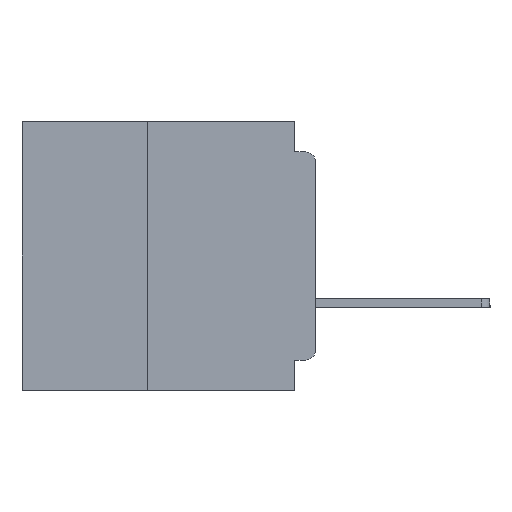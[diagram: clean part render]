
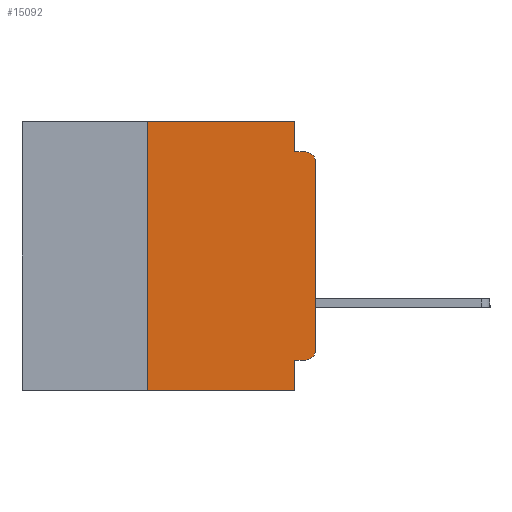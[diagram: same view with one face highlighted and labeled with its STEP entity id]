
A CAD part, left-side view. The second image highlights one B-rep face of the part: STEP entity #15092.
In plain terms, the highlighted planar face has unit normal (-1, 0, 0).
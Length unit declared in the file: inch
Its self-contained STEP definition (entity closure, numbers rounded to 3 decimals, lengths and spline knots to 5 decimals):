
#999 = VERTEX_POINT ( 'NONE', #19399 ) ;
#2351 = VECTOR ( 'NONE', #28648, 39.37008 ) ;
#2496 = EDGE_CURVE ( 'NONE', #19517, #46442, #31707, .T. ) ;
#2629 = VECTOR ( 'NONE', #43615, 39.37008 ) ;
#3094 = DIRECTION ( 'NONE',  ( 1., 0., 0. ) ) ;
#3157 = VERTEX_POINT ( 'NONE', #3941 ) ;
#3846 = DIRECTION ( 'NONE',  ( 0., -1., 0. ) ) ;
#3941 = CARTESIAN_POINT ( 'NONE',  ( 0., 0.031, -0.4 ) ) ;
#4085 = CARTESIAN_POINT ( 'NONE',  ( 0., 0.031, -0.4 ) ) ;
#4223 = CIRCLE ( 'NONE', #15329, 0.015 ) ;
#4745 = AXIS2_PLACEMENT_3D ( 'NONE', #50031, #23268, #54496 ) ;
#5116 = FACE_OUTER_BOUND ( 'NONE', #40707, .T. ) ;
#6350 = ORIENTED_EDGE ( 'NONE', *, *, #2496, .F. ) ;
#6652 = CARTESIAN_POINT ( 'NONE',  ( 0., 0.25, 0. ) ) ;
#7062 = ORIENTED_EDGE ( 'NONE', *, *, #38648, .F. ) ;
#8152 = EDGE_CURVE ( 'NONE', #999, #46442, #39294, .T. ) ;
#9086 = VERTEX_POINT ( 'NONE', #50397 ) ;
#9133 = ORIENTED_EDGE ( 'NONE', *, *, #21277, .T. ) ;
#10361 = ORIENTED_EDGE ( 'NONE', *, *, #40444, .F. ) ;
#11088 = VERTEX_POINT ( 'NONE', #11302 ) ;
#11302 = CARTESIAN_POINT ( 'NONE',  ( 0., 0.031, 0. ) ) ;
#12837 = CARTESIAN_POINT ( 'NONE',  ( 0., 0.437, -0.4 ) ) ;
#14018 = VECTOR ( 'NONE', #33196, 39.37008 ) ;
#14271 = LINE ( 'NONE', #41947, #2351 ) ;
#14731 = DIRECTION ( 'NONE',  ( 0., 0., 1. ) ) ;
#15092 = ADVANCED_FACE ( 'NONE', ( #5116 ), #25360, .F. ) ;
#15226 = CARTESIAN_POINT ( 'NONE',  ( 0., 0., -0.355 ) ) ;
#15329 = AXIS2_PLACEMENT_3D ( 'NONE', #21290, #52503, #25749 ) ;
#15903 = LINE ( 'NONE', #46033, #39646 ) ;
#18441 = VECTOR ( 'NONE', #56700, 39.37008 ) ;
#19144 = ORIENTED_EDGE ( 'NONE', *, *, #37119, .F. ) ;
#19195 = LINE ( 'NONE', #4085, #53429 ) ;
#19399 = CARTESIAN_POINT ( 'NONE',  ( 0., 0., -0.06 ) ) ;
#19517 = VERTEX_POINT ( 'NONE', #54055 ) ;
#20667 = VERTEX_POINT ( 'NONE', #41585 ) ;
#21005 = CARTESIAN_POINT ( 'NONE',  ( 0., 0., -0.045 ) ) ;
#21277 = EDGE_CURVE ( 'NONE', #20667, #999, #15903, .T. ) ;
#21290 = CARTESIAN_POINT ( 'NONE',  ( 0., 0.015, -0.34 ) ) ;
#22080 = CARTESIAN_POINT ( 'NONE',  ( 0., 0.015, -0.355 ) ) ;
#23118 = VECTOR ( 'NONE', #3846, 39.37008 ) ;
#23268 = DIRECTION ( 'NONE',  ( -1., 0., 0. ) ) ;
#25360 = PLANE ( 'NONE',  #29732 ) ;
#25749 = DIRECTION ( 'NONE',  ( 0., 0., -1. ) ) ;
#25896 = LINE ( 'NONE', #15226, #14018 ) ;
#28648 = DIRECTION ( 'NONE',  ( 0., 0., 1. ) ) ;
#28824 = VERTEX_POINT ( 'NONE', #46643 ) ;
#29732 = AXIS2_PLACEMENT_3D ( 'NONE', #56581, #3094, #34353 ) ;
#31707 = LINE ( 'NONE', #21005, #18441 ) ;
#33194 = ORIENTED_EDGE ( 'NONE', *, *, #40714, .F. ) ;
#33196 = DIRECTION ( 'NONE',  ( 0., 1., 0. ) ) ;
#33329 = DIRECTION ( 'NONE',  ( 0., -1., 0. ) ) ;
#34353 = DIRECTION ( 'NONE',  ( 0., 0., -1. ) ) ;
#34751 = LINE ( 'NONE', #55386, #45253 ) ;
#35011 = LINE ( 'NONE', #12837, #23118 ) ;
#35567 = VERTEX_POINT ( 'NONE', #6652 ) ;
#36502 = ORIENTED_EDGE ( 'NONE', *, *, #37325, .T. ) ;
#37119 = EDGE_CURVE ( 'NONE', #51397, #9086, #25896, .T. ) ;
#37325 = EDGE_CURVE ( 'NONE', #51397, #20667, #4223, .T. ) ;
#38648 = EDGE_CURVE ( 'NONE', #11088, #19517, #48793, .T. ) ;
#39294 = CIRCLE ( 'NONE', #4745, 0.015 ) ;
#39646 = VECTOR ( 'NONE', #14731, 39.37008 ) ;
#40444 = EDGE_CURVE ( 'NONE', #9086, #3157, #19195, .T. ) ;
#40707 = EDGE_LOOP ( 'NONE', ( #9133, #46106, #6350, #7062, #42243, #33194, #49596, #10361, #19144, #36502 ) ) ;
#40714 = EDGE_CURVE ( 'NONE', #28824, #35567, #14271, .T. ) ;
#41585 = CARTESIAN_POINT ( 'NONE',  ( 0., 0., -0.34 ) ) ;
#41947 = CARTESIAN_POINT ( 'NONE',  ( 0., 0.25, -0.4 ) ) ;
#42243 = ORIENTED_EDGE ( 'NONE', *, *, #42609, .F. ) ;
#42609 = EDGE_CURVE ( 'NONE', #35567, #11088, #34751, .T. ) ;
#43615 = DIRECTION ( 'NONE',  ( 0., 0., -1. ) ) ;
#45253 = VECTOR ( 'NONE', #33329, 39.37008 ) ;
#46033 = CARTESIAN_POINT ( 'NONE',  ( 0., 0., 0. ) ) ;
#46106 = ORIENTED_EDGE ( 'NONE', *, *, #8152, .T. ) ;
#46442 = VERTEX_POINT ( 'NONE', #47539 ) ;
#46643 = CARTESIAN_POINT ( 'NONE',  ( 0., 0.25, -0.4 ) ) ;
#47539 = CARTESIAN_POINT ( 'NONE',  ( 0., 0.015, -0.045 ) ) ;
#48793 = LINE ( 'NONE', #52559, #2629 ) ;
#49596 = ORIENTED_EDGE ( 'NONE', *, *, #51128, .T. ) ;
#50031 = CARTESIAN_POINT ( 'NONE',  ( 0., 0.015, -0.06 ) ) ;
#50397 = CARTESIAN_POINT ( 'NONE',  ( 0., 0.031, -0.355 ) ) ;
#51128 = EDGE_CURVE ( 'NONE', #28824, #3157, #35011, .T. ) ;
#51397 = VERTEX_POINT ( 'NONE', #22080 ) ;
#52503 = DIRECTION ( 'NONE',  ( -1., 0., 0. ) ) ;
#52559 = CARTESIAN_POINT ( 'NONE',  ( 0., 0.031, 0. ) ) ;
#53429 = VECTOR ( 'NONE', #57587, 39.37008 ) ;
#54055 = CARTESIAN_POINT ( 'NONE',  ( 0., 0.031, -0.045 ) ) ;
#54496 = DIRECTION ( 'NONE',  ( 0., 0., -1. ) ) ;
#55386 = CARTESIAN_POINT ( 'NONE',  ( 0., 0.437, 0. ) ) ;
#56581 = CARTESIAN_POINT ( 'NONE',  ( 0., 0.437, 0. ) ) ;
#56700 = DIRECTION ( 'NONE',  ( 0., -1., 0. ) ) ;
#57587 = DIRECTION ( 'NONE',  ( 0., 0., -1. ) ) ;
